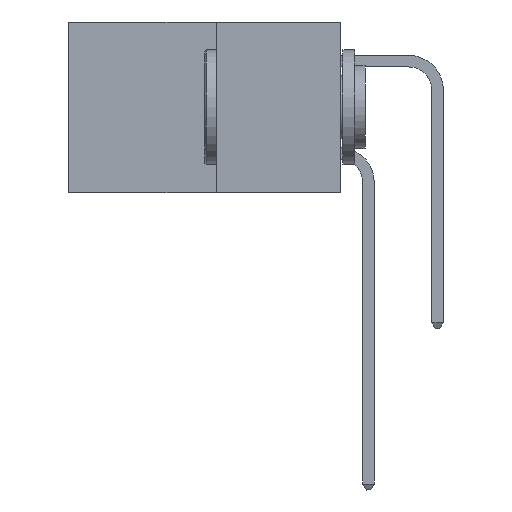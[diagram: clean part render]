
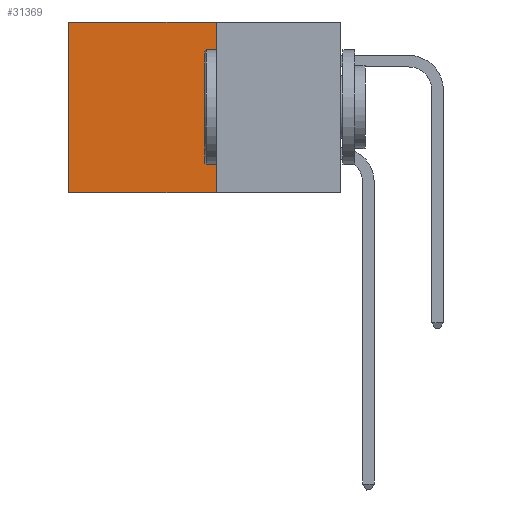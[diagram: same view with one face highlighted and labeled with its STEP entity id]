
A CAD part, left-side view. The second image highlights one B-rep face of the part: STEP entity #31369.
In plain terms, the highlighted planar face has unit normal (-1, 0, 0).
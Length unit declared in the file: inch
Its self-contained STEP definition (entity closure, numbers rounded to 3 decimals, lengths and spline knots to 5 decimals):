
#1613 = CARTESIAN_POINT ( 'NONE',  ( 0.277, 0.59, -0.37 ) ) ;
#2908 = DIRECTION ( 'NONE',  ( 1., 0., 0. ) ) ;
#3683 = VERTEX_POINT ( 'NONE', #27434 ) ;
#4736 = VECTOR ( 'NONE', #18357, 39.37008 ) ;
#6794 = DIRECTION ( 'NONE',  ( 0., 0., -1. ) ) ;
#6884 = CARTESIAN_POINT ( 'NONE',  ( 0.277, 0.27, -0.37 ) ) ;
#8229 = LINE ( 'NONE', #21056, #22551 ) ;
#9117 = LINE ( 'NONE', #28783, #22543 ) ;
#9730 = CARTESIAN_POINT ( 'NONE',  ( 0.277, 0.27, 0. ) ) ;
#11055 = ORIENTED_EDGE ( 'NONE', *, *, #33506, .F. ) ;
#11752 = ORIENTED_EDGE ( 'NONE', *, *, #25781, .T. ) ;
#15583 = ORIENTED_EDGE ( 'NONE', *, *, #24751, .T. ) ;
#18357 = DIRECTION ( 'NONE',  ( 0., 1., 0. ) ) ;
#20421 = VERTEX_POINT ( 'NONE', #36482 ) ;
#21056 = CARTESIAN_POINT ( 'NONE',  ( 0.277, 0.27, -0.37 ) ) ;
#22543 = VECTOR ( 'NONE', #31662, 39.37008 ) ;
#22551 = VECTOR ( 'NONE', #6794, 39.37008 ) ;
#22926 = DIRECTION ( 'NONE',  ( 0., 0., -1. ) ) ;
#24751 = EDGE_CURVE ( 'NONE', #34628, #3683, #34680, .T. ) ;
#25781 = EDGE_CURVE ( 'NONE', #30286, #34628, #9117, .T. ) ;
#27073 = VECTOR ( 'NONE', #32965, 39.37008 ) ;
#27434 = CARTESIAN_POINT ( 'NONE',  ( 0.277, 0.59, -0.37 ) ) ;
#28531 = CARTESIAN_POINT ( 'NONE',  ( 0.277, 0.27, -0.37 ) ) ;
#28783 = CARTESIAN_POINT ( 'NONE',  ( 0.277, 0.27, 0. ) ) ;
#28956 = CARTESIAN_POINT ( 'NONE',  ( 0.277, 0.59, 0. ) ) ;
#29549 = AXIS2_PLACEMENT_3D ( 'NONE', #28531, #2908, #22926 ) ;
#30286 = VERTEX_POINT ( 'NONE', #9730 ) ;
#30304 = FACE_OUTER_BOUND ( 'NONE', #30370, .T. ) ;
#30370 = EDGE_LOOP ( 'NONE', ( #15583, #31939, #11055, #11752 ) ) ;
#31369 = ADVANCED_FACE ( 'NONE', ( #30304 ), #34273, .F. ) ;
#31662 = DIRECTION ( 'NONE',  ( 0., 1., 0. ) ) ;
#31939 = ORIENTED_EDGE ( 'NONE', *, *, #32281, .F. ) ;
#32281 = EDGE_CURVE ( 'NONE', #20421, #3683, #36057, .T. ) ;
#32965 = DIRECTION ( 'NONE',  ( 0., 0., -1. ) ) ;
#33506 = EDGE_CURVE ( 'NONE', #30286, #20421, #8229, .T. ) ;
#34273 = PLANE ( 'NONE',  #29549 ) ;
#34628 = VERTEX_POINT ( 'NONE', #28956 ) ;
#34680 = LINE ( 'NONE', #1613, #27073 ) ;
#36057 = LINE ( 'NONE', #6884, #4736 ) ;
#36482 = CARTESIAN_POINT ( 'NONE',  ( 0.277, 0.27, -0.37 ) ) ;
